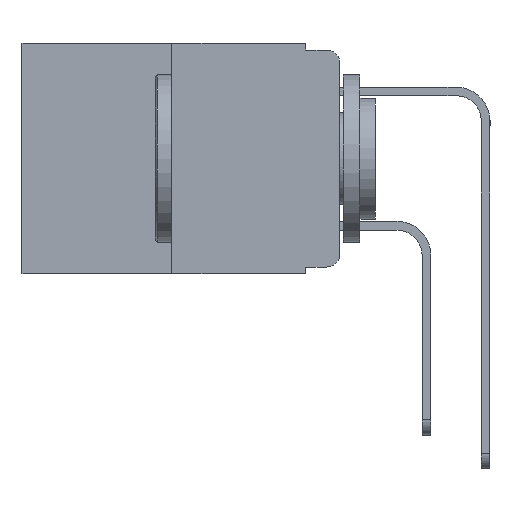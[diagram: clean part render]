
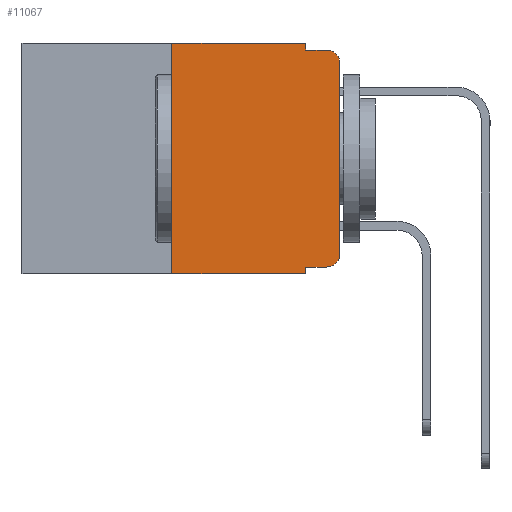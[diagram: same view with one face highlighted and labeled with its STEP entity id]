
A CAD part, left-side view. The second image highlights one B-rep face of the part: STEP entity #11067.
In plain terms, the highlighted planar face has unit normal (-1, 0, 0).
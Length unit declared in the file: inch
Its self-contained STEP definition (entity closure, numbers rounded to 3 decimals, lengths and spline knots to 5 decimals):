
#10 = VERTEX_POINT ( 'NONE', #1022 ) ;
#354 = AXIS2_PLACEMENT_3D ( 'NONE', #9440, #495, #10892 ) ;
#495 = DIRECTION ( 'NONE',  ( -1., 0., 0. ) ) ;
#683 = DIRECTION ( 'NONE',  ( 1., 0., 0. ) ) ;
#1022 = CARTESIAN_POINT ( 'NONE',  ( 0., 0.051, -0.343 ) ) ;
#1045 = ORIENTED_EDGE ( 'NONE', *, *, #9703, .T. ) ;
#1156 = VECTOR ( 'NONE', #3854, 39.37008 ) ;
#1252 = ORIENTED_EDGE ( 'NONE', *, *, #9963, .F. ) ;
#1299 = ORIENTED_EDGE ( 'NONE', *, *, #9970, .F. ) ;
#2103 = VECTOR ( 'NONE', #11014, 39.37008 ) ;
#2134 = CARTESIAN_POINT ( 'NONE',  ( 0., 0.051, 0. ) ) ;
#2548 = VERTEX_POINT ( 'NONE', #16064 ) ;
#2836 = ORIENTED_EDGE ( 'NONE', *, *, #9994, .T. ) ;
#3579 = CIRCLE ( 'NONE', #354, 0.02 ) ;
#3705 = DIRECTION ( 'NONE',  ( 0., 0., -1. ) ) ;
#3782 = VERTEX_POINT ( 'NONE', #7362 ) ;
#3815 = VERTEX_POINT ( 'NONE', #4546 ) ;
#3854 = DIRECTION ( 'NONE',  ( 0., -1., 0. ) ) ;
#4546 = CARTESIAN_POINT ( 'NONE',  ( 0., 0.051, -0.01 ) ) ;
#5015 = ORIENTED_EDGE ( 'NONE', *, *, #9943, .T. ) ;
#5081 = DIRECTION ( 'NONE',  ( 0., -1., 0. ) ) ;
#5203 = CARTESIAN_POINT ( 'NONE',  ( 0., 0.02, -0.313 ) ) ;
#5431 = AXIS2_PLACEMENT_3D ( 'NONE', #5203, #15347, #6737 ) ;
#5623 = LINE ( 'NONE', #16846, #1156 ) ;
#5725 = CARTESIAN_POINT ( 'NONE',  ( 0., 0.051, 0. ) ) ;
#6366 = ORIENTED_EDGE ( 'NONE', *, *, #9939, .T. ) ;
#6569 = VECTOR ( 'NONE', #10960, 39.37008 ) ;
#6737 = DIRECTION ( 'NONE',  ( 0., 0., -1. ) ) ;
#7041 = LINE ( 'NONE', #16593, #15147 ) ;
#7251 = DIRECTION ( 'NONE',  ( 0., -1., 0. ) ) ;
#7362 = CARTESIAN_POINT ( 'NONE',  ( 0., 0.02, -0.01 ) ) ;
#7527 = VERTEX_POINT ( 'NONE', #17770 ) ;
#8035 = VERTEX_POINT ( 'NONE', #10720 ) ;
#9267 = AXIS2_PLACEMENT_3D ( 'NONE', #15334, #683, #11059 ) ;
#9315 = EDGE_CURVE ( 'NONE', #16592, #16074, #16295, .T. ) ;
#9440 = CARTESIAN_POINT ( 'NONE',  ( 0., 0.02, -0.03 ) ) ;
#9500 = CARTESIAN_POINT ( 'NONE',  ( 0., 0.25, 0. ) ) ;
#9703 = EDGE_CURVE ( 'NONE', #11792, #10, #5623, .T. ) ;
#9939 = EDGE_CURVE ( 'NONE', #8035, #7527, #11776, .T. ) ;
#9943 = EDGE_CURVE ( 'NONE', #7527, #3782, #3579, .T. ) ;
#9951 = CIRCLE ( 'NONE', #5431, 0.02 ) ;
#9963 = EDGE_CURVE ( 'NONE', #3815, #3782, #7041, .T. ) ;
#9965 = EDGE_CURVE ( 'NONE', #16074, #3815, #14698, .T. ) ;
#9968 = EDGE_CURVE ( 'NONE', #11792, #16592, #17908, .T. ) ;
#9970 = EDGE_CURVE ( 'NONE', #2548, #10, #10408, .T. ) ;
#9994 = EDGE_CURVE ( 'NONE', #2548, #18430, #13788, .T. ) ;
#9999 = EDGE_CURVE ( 'NONE', #18430, #8035, #9951, .T. ) ;
#10408 = LINE ( 'NONE', #2134, #17505 ) ;
#10720 = CARTESIAN_POINT ( 'NONE',  ( 0., 0., -0.313 ) ) ;
#10892 = DIRECTION ( 'NONE',  ( 0., 0., -1. ) ) ;
#10960 = DIRECTION ( 'NONE',  ( 0., 0., 1. ) ) ;
#11014 = DIRECTION ( 'NONE',  ( 0., -1., 0. ) ) ;
#11059 = DIRECTION ( 'NONE',  ( 0., 0., -1. ) ) ;
#11067 = ADVANCED_FACE ( 'NONE', ( #12387 ), #12450, .F. ) ;
#11204 = ORIENTED_EDGE ( 'NONE', *, *, #9999, .T. ) ;
#11520 = ORIENTED_EDGE ( 'NONE', *, *, #9315, .F. ) ;
#11654 = ORIENTED_EDGE ( 'NONE', *, *, #9965, .F. ) ;
#11776 = LINE ( 'NONE', #17857, #18310 ) ;
#11792 = VERTEX_POINT ( 'NONE', #14691 ) ;
#12375 = ORIENTED_EDGE ( 'NONE', *, *, #9968, .F. ) ;
#12387 = FACE_OUTER_BOUND ( 'NONE', #12895, .T. ) ;
#12450 = PLANE ( 'NONE',  #9267 ) ;
#12473 = VECTOR ( 'NONE', #7251, 39.37008 ) ;
#12840 = CARTESIAN_POINT ( 'NONE',  ( 0., 0.25, 0. ) ) ;
#12895 = EDGE_LOOP ( 'NONE', ( #6366, #5015, #1252, #11654, #11520, #12375, #1045, #1299, #2836, #11204 ) ) ;
#12990 = CARTESIAN_POINT ( 'NONE',  ( 0., 0.473, 0. ) ) ;
#13788 = LINE ( 'NONE', #18024, #2103 ) ;
#14238 = VECTOR ( 'NONE', #17960, 39.37008 ) ;
#14691 = CARTESIAN_POINT ( 'NONE',  ( 0., 0.25, -0.343 ) ) ;
#14698 = LINE ( 'NONE', #16641, #14238 ) ;
#15147 = VECTOR ( 'NONE', #5081, 39.37008 ) ;
#15175 = DIRECTION ( 'NONE',  ( 0., 0., 1. ) ) ;
#15334 = CARTESIAN_POINT ( 'NONE',  ( 0., 0.473, 0. ) ) ;
#15347 = DIRECTION ( 'NONE',  ( -1., 0., 0. ) ) ;
#16064 = CARTESIAN_POINT ( 'NONE',  ( 0., 0.051, -0.333 ) ) ;
#16074 = VERTEX_POINT ( 'NONE', #5725 ) ;
#16295 = LINE ( 'NONE', #12990, #12473 ) ;
#16592 = VERTEX_POINT ( 'NONE', #12840 ) ;
#16593 = CARTESIAN_POINT ( 'NONE',  ( 0., 0.051, -0.01 ) ) ;
#16641 = CARTESIAN_POINT ( 'NONE',  ( 0., 0.051, 0. ) ) ;
#16846 = CARTESIAN_POINT ( 'NONE',  ( 0., 0.473, -0.343 ) ) ;
#17505 = VECTOR ( 'NONE', #3705, 39.37008 ) ;
#17770 = CARTESIAN_POINT ( 'NONE',  ( 0., 0., -0.03 ) ) ;
#17857 = CARTESIAN_POINT ( 'NONE',  ( 0., 0., 0. ) ) ;
#17908 = LINE ( 'NONE', #9500, #6569 ) ;
#17960 = DIRECTION ( 'NONE',  ( 0., 0., -1. ) ) ;
#18024 = CARTESIAN_POINT ( 'NONE',  ( 0., 0.051, -0.333 ) ) ;
#18310 = VECTOR ( 'NONE', #15175, 39.37008 ) ;
#18430 = VERTEX_POINT ( 'NONE', #18709 ) ;
#18709 = CARTESIAN_POINT ( 'NONE',  ( 0., 0.02, -0.333 ) ) ;
